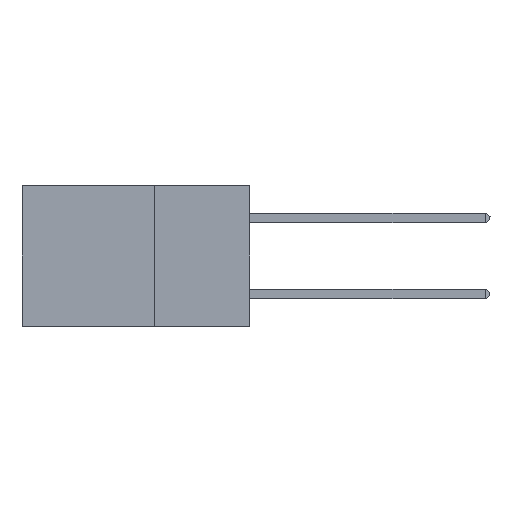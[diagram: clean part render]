
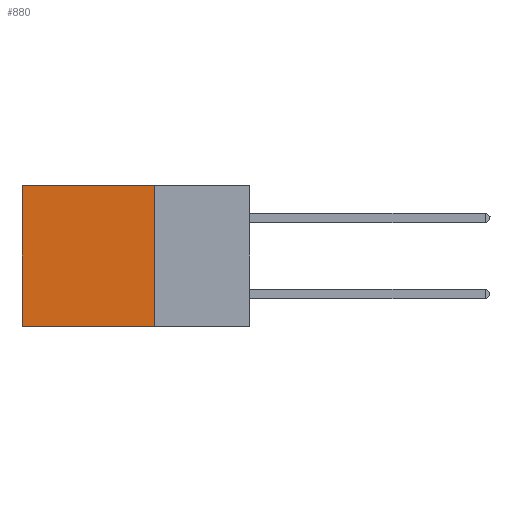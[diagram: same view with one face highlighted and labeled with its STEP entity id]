
A CAD part, left-side view. The second image highlights one B-rep face of the part: STEP entity #880.
In plain terms, the highlighted planar face has unit normal (-1, 0, 0).
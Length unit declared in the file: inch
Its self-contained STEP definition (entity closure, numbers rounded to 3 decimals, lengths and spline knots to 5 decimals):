
#880 = ADVANCED_FACE ( 'NONE', ( #2203 ), #11065, .F. ) ;
#919 = CARTESIAN_POINT ( 'NONE',  ( 0.2875, 0.25, 0. ) ) ;
#1107 = VERTEX_POINT ( 'NONE', #9139 ) ;
#1760 = CARTESIAN_POINT ( 'NONE',  ( 0.2875, 0.25, 0. ) ) ;
#2203 = FACE_OUTER_BOUND ( 'NONE', #11343, .T. ) ;
#2543 = ORIENTED_EDGE ( 'NONE', *, *, #8011, .F. ) ;
#2713 = EDGE_CURVE ( 'NONE', #10002, #17863, #4981, .T. ) ;
#2942 = DIRECTION ( 'NONE',  ( 0., 1., 0. ) ) ;
#3224 = ORIENTED_EDGE ( 'NONE', *, *, #6749, .T. ) ;
#3429 = EDGE_CURVE ( 'NONE', #13309, #17863, #12881, .T. ) ;
#3507 = AXIS2_PLACEMENT_3D ( 'NONE', #1760, #6528, #12537 ) ;
#4585 = CARTESIAN_POINT ( 'NONE',  ( 0.2875, 0.25, -0.37 ) ) ;
#4706 = ORIENTED_EDGE ( 'NONE', *, *, #2713, .T. ) ;
#4731 = CARTESIAN_POINT ( 'NONE',  ( 0.2875, 0.6, -0.37 ) ) ;
#4981 = LINE ( 'NONE', #17762, #6189 ) ;
#5847 = ORIENTED_EDGE ( 'NONE', *, *, #3429, .F. ) ;
#6189 = VECTOR ( 'NONE', #14799, 39.37008 ) ;
#6193 = VECTOR ( 'NONE', #10067, 39.37008 ) ;
#6528 = DIRECTION ( 'NONE',  ( 1., 0., 0. ) ) ;
#6749 = EDGE_CURVE ( 'NONE', #1107, #10002, #11543, .T. ) ;
#6937 = CARTESIAN_POINT ( 'NONE',  ( 0.2875, 0.6, 0. ) ) ;
#8011 = EDGE_CURVE ( 'NONE', #1107, #13309, #18495, .T. ) ;
#9139 = CARTESIAN_POINT ( 'NONE',  ( 0.2875, 0.25, 0. ) ) ;
#10002 = VERTEX_POINT ( 'NONE', #6937 ) ;
#10067 = DIRECTION ( 'NONE',  ( 0., 1., 0. ) ) ;
#10788 = VECTOR ( 'NONE', #11690, 39.37008 ) ;
#11065 = PLANE ( 'NONE',  #3507 ) ;
#11343 = EDGE_LOOP ( 'NONE', ( #4706, #5847, #2543, #3224 ) ) ;
#11543 = LINE ( 'NONE', #12079, #12984 ) ;
#11690 = DIRECTION ( 'NONE',  ( 0., 0., -1. ) ) ;
#12079 = CARTESIAN_POINT ( 'NONE',  ( 0.2875, 0.25, 0. ) ) ;
#12537 = DIRECTION ( 'NONE',  ( 0., 0., -1. ) ) ;
#12881 = LINE ( 'NONE', #17341, #6193 ) ;
#12984 = VECTOR ( 'NONE', #2942, 39.37008 ) ;
#13309 = VERTEX_POINT ( 'NONE', #4585 ) ;
#14799 = DIRECTION ( 'NONE',  ( 0., 0., -1. ) ) ;
#17341 = CARTESIAN_POINT ( 'NONE',  ( 0.2875, 0.25, -0.37 ) ) ;
#17762 = CARTESIAN_POINT ( 'NONE',  ( 0.2875, 0.6, 0. ) ) ;
#17863 = VERTEX_POINT ( 'NONE', #4731 ) ;
#18495 = LINE ( 'NONE', #919, #10788 ) ;
